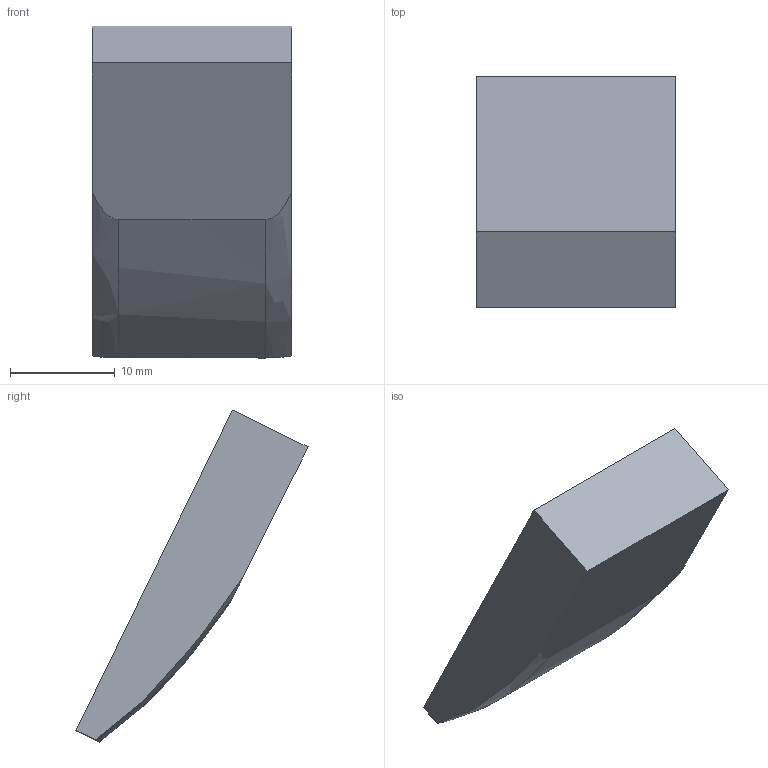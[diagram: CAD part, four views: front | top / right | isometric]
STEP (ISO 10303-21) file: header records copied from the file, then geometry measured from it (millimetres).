
FILE_DESCRIPTION((''),'2;1');
FILE_NAME('PM422FrameCap1.stp','2015-05-13T23:48:34',('JamesRPatrick'),(''),'Autodesk Inventor 2012','Autodesk Inventor 2012','');
FILE_SCHEMA(('AUTOMOTIVE_DESIGN { 1 0 10303 214 1 1 1 1 }'));
Length unit declared in the file: millimetre
Products named in the file (1): PM422FrameCap1
Bounding box: 19 x 22.13 x 31.66 mm (x, y, z)
Volume: 4402.9 mm3; surface area: 1959.6 mm2
Topology: 1 solids, 1 shells, 9 faces, 22 edges, 15 vertices
Faces by surface type: plane 6, bspline 3
Entity records: 401 total; most frequent: CARTESIAN_POINT 185, ORIENTED_EDGE 44, DIRECTION 27, EDGE_CURVE 22, VERTEX_POINT 15, VECTOR 13, LINE 13, EDGE_LOOP 9
